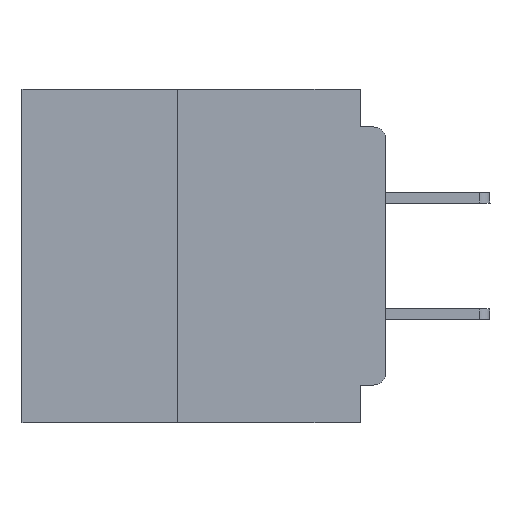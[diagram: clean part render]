
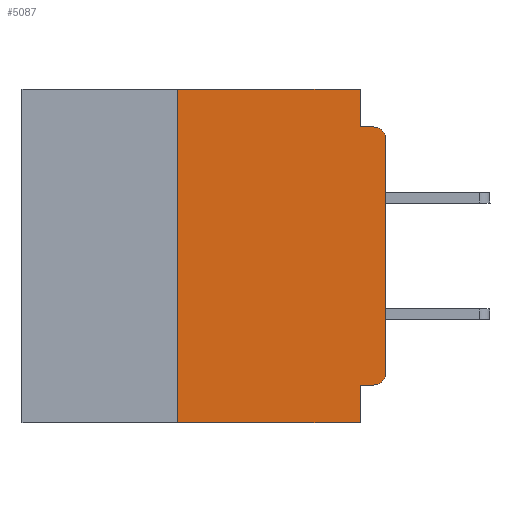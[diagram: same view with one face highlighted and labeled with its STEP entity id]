
A CAD part, left-side view. The second image highlights one B-rep face of the part: STEP entity #5087.
In plain terms, the highlighted planar face has unit normal (-1, 0, 0).
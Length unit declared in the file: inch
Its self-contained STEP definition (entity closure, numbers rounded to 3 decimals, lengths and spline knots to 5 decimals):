
#476 = EDGE_CURVE ( 'NONE', #25719, #37187, #16884, .T. ) ;
#796 = DIRECTION ( 'NONE',  ( -1., 0., 0. ) ) ;
#1408 = ORIENTED_EDGE ( 'NONE', *, *, #43257, .F. ) ;
#3674 = DIRECTION ( 'NONE',  ( 0., -1., 0. ) ) ;
#5087 = ADVANCED_FACE ( 'NONE', ( #35687 ), #42963, .F. ) ;
#5129 = VECTOR ( 'NONE', #51685, 39.37008 ) ;
#6634 = CARTESIAN_POINT ( 'NONE',  ( 0., 0.015, -0.34 ) ) ;
#7046 = CARTESIAN_POINT ( 'NONE',  ( 0., 0.437, 0. ) ) ;
#7391 = ORIENTED_EDGE ( 'NONE', *, *, #31839, .F. ) ;
#7539 = CARTESIAN_POINT ( 'NONE',  ( 0., 0., 0. ) ) ;
#7560 = VECTOR ( 'NONE', #3674, 39.37008 ) ;
#7971 = VECTOR ( 'NONE', #59519, 39.37008 ) ;
#8746 = CARTESIAN_POINT ( 'NONE',  ( 0., 0., -0.045 ) ) ;
#9941 = ORIENTED_EDGE ( 'NONE', *, *, #20569, .F. ) ;
#11756 = DIRECTION ( 'NONE',  ( 0., 0., -1. ) ) ;
#12276 = DIRECTION ( 'NONE',  ( 1., 0., 0. ) ) ;
#13712 = VERTEX_POINT ( 'NONE', #13799 ) ;
#13799 = CARTESIAN_POINT ( 'NONE',  ( 0., 0.031, -0.4 ) ) ;
#13968 = AXIS2_PLACEMENT_3D ( 'NONE', #47817, #12276, #48038 ) ;
#14628 = VECTOR ( 'NONE', #16316, 39.37008 ) ;
#15117 = CARTESIAN_POINT ( 'NONE',  ( 0., 0., -0.34 ) ) ;
#15986 = CARTESIAN_POINT ( 'NONE',  ( 0., 0.015, -0.355 ) ) ;
#16316 = DIRECTION ( 'NONE',  ( 0., 0., 1. ) ) ;
#16884 = LINE ( 'NONE', #7539, #42517 ) ;
#18332 = CARTESIAN_POINT ( 'NONE',  ( 0., 0.25, 0. ) ) ;
#18551 = ORIENTED_EDGE ( 'NONE', *, *, #25376, .T. ) ;
#18598 = VECTOR ( 'NONE', #34080, 39.37008 ) ;
#18708 = LINE ( 'NONE', #56773, #5129 ) ;
#18780 = VECTOR ( 'NONE', #22246, 39.37008 ) ;
#19076 = CARTESIAN_POINT ( 'NONE',  ( 0., 0.015, -0.045 ) ) ;
#20569 = EDGE_CURVE ( 'NONE', #63037, #53873, #59436, .T. ) ;
#21527 = DIRECTION ( 'NONE',  ( 0., 0., -1. ) ) ;
#21581 = LINE ( 'NONE', #54226, #7971 ) ;
#22246 = DIRECTION ( 'NONE',  ( 0., -1., 0. ) ) ;
#22436 = EDGE_CURVE ( 'NONE', #35470, #63037, #41863, .T. ) ;
#23597 = AXIS2_PLACEMENT_3D ( 'NONE', #6634, #42420, #11756 ) ;
#25376 = EDGE_CURVE ( 'NONE', #30068, #25719, #66001, .T. ) ;
#25719 = VERTEX_POINT ( 'NONE', #15117 ) ;
#26659 = VERTEX_POINT ( 'NONE', #63073 ) ;
#28104 = EDGE_CURVE ( 'NONE', #26659, #41492, #48367, .T. ) ;
#30068 = VERTEX_POINT ( 'NONE', #15986 ) ;
#31278 = CARTESIAN_POINT ( 'NONE',  ( 0., 0.25, -0.4 ) ) ;
#31367 = CARTESIAN_POINT ( 'NONE',  ( 0., 0.015, -0.06 ) ) ;
#31839 = EDGE_CURVE ( 'NONE', #46084, #13712, #64556, .T. ) ;
#32192 = LINE ( 'NONE', #44372, #18598 ) ;
#34080 = DIRECTION ( 'NONE',  ( 0., 1., 0. ) ) ;
#35470 = VERTEX_POINT ( 'NONE', #43427 ) ;
#35687 = FACE_OUTER_BOUND ( 'NONE', #62876, .T. ) ;
#36396 = ORIENTED_EDGE ( 'NONE', *, *, #22436, .F. ) ;
#36522 = DIRECTION ( 'NONE',  ( 0., 0., -1. ) ) ;
#37187 = VERTEX_POINT ( 'NONE', #53217 ) ;
#37900 = ORIENTED_EDGE ( 'NONE', *, *, #28104, .F. ) ;
#39046 = ORIENTED_EDGE ( 'NONE', *, *, #60020, .F. ) ;
#41088 = EDGE_CURVE ( 'NONE', #35470, #13712, #18708, .T. ) ;
#41492 = VERTEX_POINT ( 'NONE', #19076 ) ;
#41863 = LINE ( 'NONE', #31278, #14628 ) ;
#42420 = DIRECTION ( 'NONE',  ( -1., 0., 0. ) ) ;
#42517 = VECTOR ( 'NONE', #53526, 39.37008 ) ;
#42963 = PLANE ( 'NONE',  #13968 ) ;
#43257 = EDGE_CURVE ( 'NONE', #53873, #26659, #21581, .T. ) ;
#43427 = CARTESIAN_POINT ( 'NONE',  ( 0., 0.25, -0.4 ) ) ;
#44222 = EDGE_CURVE ( 'NONE', #37187, #41492, #58464, .T. ) ;
#44372 = CARTESIAN_POINT ( 'NONE',  ( 0., 0., -0.355 ) ) ;
#45676 = CARTESIAN_POINT ( 'NONE',  ( 0., 0.031, 0. ) ) ;
#46084 = VERTEX_POINT ( 'NONE', #48269 ) ;
#47817 = CARTESIAN_POINT ( 'NONE',  ( 0., 0.437, 0. ) ) ;
#47935 = VECTOR ( 'NONE', #21527, 39.37008 ) ;
#48038 = DIRECTION ( 'NONE',  ( 0., 0., -1. ) ) ;
#48269 = CARTESIAN_POINT ( 'NONE',  ( 0., 0.031, -0.355 ) ) ;
#48367 = LINE ( 'NONE', #8746, #7560 ) ;
#50375 = AXIS2_PLACEMENT_3D ( 'NONE', #31367, #796, #36522 ) ;
#51685 = DIRECTION ( 'NONE',  ( 0., -1., 0. ) ) ;
#52982 = ORIENTED_EDGE ( 'NONE', *, *, #41088, .T. ) ;
#53217 = CARTESIAN_POINT ( 'NONE',  ( 0., 0., -0.06 ) ) ;
#53526 = DIRECTION ( 'NONE',  ( 0., 0., 1. ) ) ;
#53873 = VERTEX_POINT ( 'NONE', #45676 ) ;
#54226 = CARTESIAN_POINT ( 'NONE',  ( 0., 0.031, 0. ) ) ;
#56773 = CARTESIAN_POINT ( 'NONE',  ( 0., 0.437, -0.4 ) ) ;
#57184 = CARTESIAN_POINT ( 'NONE',  ( 0., 0.031, -0.4 ) ) ;
#58464 = CIRCLE ( 'NONE', #50375, 0.015 ) ;
#58835 = ORIENTED_EDGE ( 'NONE', *, *, #476, .T. ) ;
#58994 = ORIENTED_EDGE ( 'NONE', *, *, #44222, .T. ) ;
#59436 = LINE ( 'NONE', #7046, #18780 ) ;
#59519 = DIRECTION ( 'NONE',  ( 0., 0., -1. ) ) ;
#60020 = EDGE_CURVE ( 'NONE', #30068, #46084, #32192, .T. ) ;
#62876 = EDGE_LOOP ( 'NONE', ( #58835, #58994, #37900, #1408, #9941, #36396, #52982, #7391, #39046, #18551 ) ) ;
#63037 = VERTEX_POINT ( 'NONE', #18332 ) ;
#63073 = CARTESIAN_POINT ( 'NONE',  ( 0., 0.031, -0.045 ) ) ;
#64556 = LINE ( 'NONE', #57184, #47935 ) ;
#66001 = CIRCLE ( 'NONE', #23597, 0.015 ) ;
